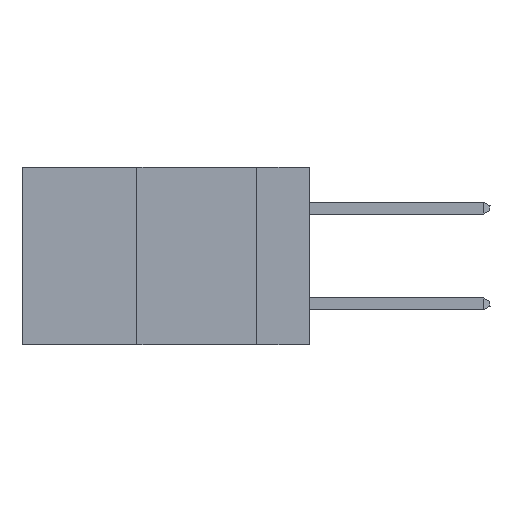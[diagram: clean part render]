
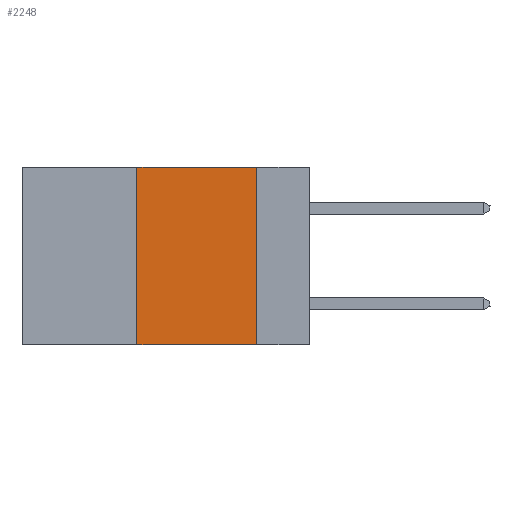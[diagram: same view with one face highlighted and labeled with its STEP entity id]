
A CAD part, left-side view. The second image highlights one B-rep face of the part: STEP entity #2248.
In plain terms, the highlighted planar face has unit normal (-1, 0, 0).
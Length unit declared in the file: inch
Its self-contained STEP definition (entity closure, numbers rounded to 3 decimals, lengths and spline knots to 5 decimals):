
#97 = VERTEX_POINT ( 'NONE', #41660 ) ;
#2248 = ADVANCED_FACE ( 'NONE', ( #14144 ), #32735, .F. ) ;
#2264 = VERTEX_POINT ( 'NONE', #10904 ) ;
#3783 = DIRECTION ( 'NONE',  ( 0., -1., 0. ) ) ;
#4266 = CARTESIAN_POINT ( 'NONE',  ( 0., 0.6, -0.37 ) ) ;
#4329 = EDGE_CURVE ( 'NONE', #2264, #33779, #34117, .T. ) ;
#8403 = EDGE_CURVE ( 'NONE', #97, #33779, #30243, .T. ) ;
#9429 = ORIENTED_EDGE ( 'NONE', *, *, #8403, .T. ) ;
#10600 = DIRECTION ( 'NONE',  ( 0., 0., 1. ) ) ;
#10904 = CARTESIAN_POINT ( 'NONE',  ( 0., 0.11, 0. ) ) ;
#11202 = AXIS2_PLACEMENT_3D ( 'NONE', #26118, #32899, #18495 ) ;
#14144 = FACE_OUTER_BOUND ( 'NONE', #22759, .T. ) ;
#15754 = DIRECTION ( 'NONE',  ( 0., -1., 0. ) ) ;
#18495 = DIRECTION ( 'NONE',  ( 0., 0., -1. ) ) ;
#18919 = CARTESIAN_POINT ( 'NONE',  ( 0., 0.11, 0. ) ) ;
#20450 = VECTOR ( 'NONE', #15754, 39.37008 ) ;
#20789 = ORIENTED_EDGE ( 'NONE', *, *, #33713, .F. ) ;
#22759 = EDGE_LOOP ( 'NONE', ( #47081, #20789, #40201, #9429 ) ) ;
#22811 = DIRECTION ( 'NONE',  ( 0., 0., -1. ) ) ;
#22836 = LINE ( 'NONE', #32755, #39622 ) ;
#26118 = CARTESIAN_POINT ( 'NONE',  ( 0., 0.6, 0. ) ) ;
#26635 = VECTOR ( 'NONE', #22811, 39.37008 ) ;
#30243 = LINE ( 'NONE', #4266, #31393 ) ;
#30710 = CARTESIAN_POINT ( 'NONE',  ( 0., 0.6, 0. ) ) ;
#31185 = CARTESIAN_POINT ( 'NONE',  ( 0., 0.11, -0.37 ) ) ;
#31393 = VECTOR ( 'NONE', #3783, 39.37008 ) ;
#32439 = CARTESIAN_POINT ( 'NONE',  ( 0., 0.36, 0. ) ) ;
#32735 = PLANE ( 'NONE',  #11202 ) ;
#32755 = CARTESIAN_POINT ( 'NONE',  ( 0., 0.36, 0. ) ) ;
#32899 = DIRECTION ( 'NONE',  ( 1., 0., 0. ) ) ;
#33177 = LINE ( 'NONE', #30710, #20450 ) ;
#33713 = EDGE_CURVE ( 'NONE', #42801, #2264, #33177, .T. ) ;
#33779 = VERTEX_POINT ( 'NONE', #31185 ) ;
#34117 = LINE ( 'NONE', #18919, #26635 ) ;
#39622 = VECTOR ( 'NONE', #10600, 39.37008 ) ;
#40201 = ORIENTED_EDGE ( 'NONE', *, *, #47254, .F. ) ;
#41660 = CARTESIAN_POINT ( 'NONE',  ( 0., 0.36, -0.37 ) ) ;
#42801 = VERTEX_POINT ( 'NONE', #32439 ) ;
#47081 = ORIENTED_EDGE ( 'NONE', *, *, #4329, .F. ) ;
#47254 = EDGE_CURVE ( 'NONE', #97, #42801, #22836, .T. ) ;
